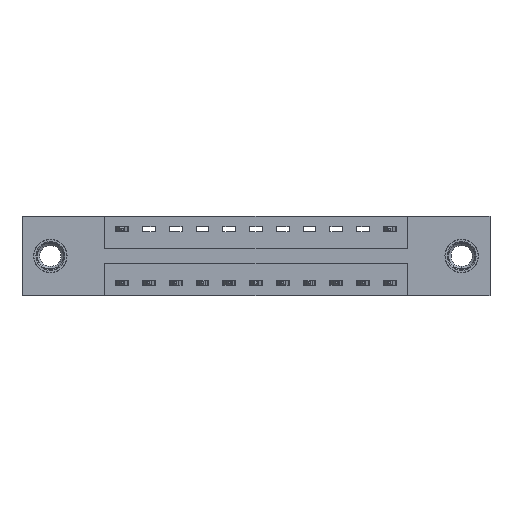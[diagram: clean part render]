
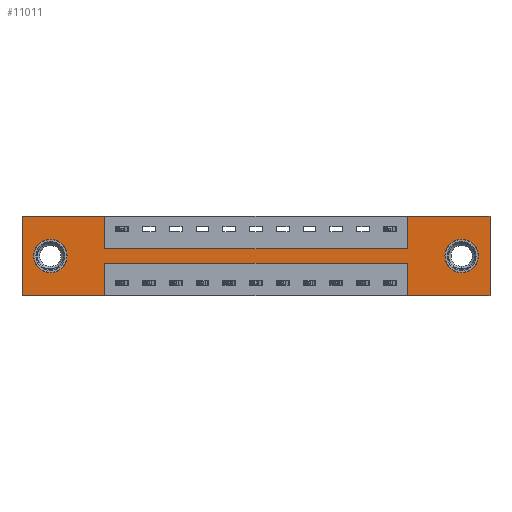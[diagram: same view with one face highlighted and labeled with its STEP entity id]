
A CAD part, front view. The second image highlights one B-rep face of the part: STEP entity #11011.
In plain terms, the highlighted planar face has unit normal (0, -1, 0).
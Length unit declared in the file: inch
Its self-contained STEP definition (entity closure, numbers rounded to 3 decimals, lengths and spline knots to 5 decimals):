
#6 = VECTOR ( 'NONE', #2793, 39.37008 ) ;
#59 = VERTEX_POINT ( 'NONE', #8711 ) ;
#99 = VERTEX_POINT ( 'NONE', #3134 ) ;
#326 = CARTESIAN_POINT ( 'NONE',  ( 0.3875, 0., -0.37 ) ) ;
#613 = VECTOR ( 'NONE', #11234, 39.37008 ) ;
#619 = VERTEX_POINT ( 'NONE', #6889 ) ;
#634 = CARTESIAN_POINT ( 'NONE',  ( 0.3875, 0., -0.15 ) ) ;
#767 = VECTOR ( 'NONE', #6159, 39.37008 ) ;
#859 = VERTEX_POINT ( 'NONE', #8142 ) ;
#861 = VECTOR ( 'NONE', #5536, 39.37008 ) ;
#1029 = CARTESIAN_POINT ( 'NONE',  ( 0.3875, 0., -0.37 ) ) ;
#1078 = VECTOR ( 'NONE', #11144, 39.37008 ) ;
#1171 = LINE ( 'NONE', #4607, #861 ) ;
#1278 = EDGE_CURVE ( 'NONE', #5420, #1296, #7348, .T. ) ;
#1296 = VERTEX_POINT ( 'NONE', #7767 ) ;
#1376 = FACE_BOUND ( 'NONE', #5382, .T. ) ;
#1487 = CIRCLE ( 'NONE', #11103, 0.078 ) ;
#1772 = CARTESIAN_POINT ( 'NONE',  ( 0.3875, 0., -0.22 ) ) ;
#1794 = LINE ( 'NONE', #8426, #11575 ) ;
#2146 = CARTESIAN_POINT ( 'NONE',  ( 2.0525, 0., -0.185 ) ) ;
#2613 = DIRECTION ( 'NONE',  ( 1., 0., 0. ) ) ;
#2614 = VECTOR ( 'NONE', #3877, 39.37008 ) ;
#2634 = VERTEX_POINT ( 'NONE', #5262 ) ;
#2656 = DIRECTION ( 'NONE',  ( 0., 1., 0. ) ) ;
#2790 = DIRECTION ( 'NONE',  ( 0., 0., 1. ) ) ;
#2793 = DIRECTION ( 'NONE',  ( -1., 0., 0. ) ) ;
#2811 = DIRECTION ( 'NONE',  ( 0., 0., 1. ) ) ;
#3043 = EDGE_LOOP ( 'NONE', ( #6996, #6897 ) ) ;
#3106 = DIRECTION ( 'NONE',  ( 0., 0., -1. ) ) ;
#3134 = CARTESIAN_POINT ( 'NONE',  ( 1.7975, 0., -0.15 ) ) ;
#3207 = LINE ( 'NONE', #10303, #613 ) ;
#3295 = EDGE_CURVE ( 'NONE', #4076, #99, #3652, .T. ) ;
#3652 = LINE ( 'NONE', #634, #5839 ) ;
#3877 = DIRECTION ( 'NONE',  ( 1., 0., 0. ) ) ;
#3961 = FACE_OUTER_BOUND ( 'NONE', #4950, .T. ) ;
#3971 = DIRECTION ( 'NONE',  ( 0., 0., -1. ) ) ;
#4076 = VERTEX_POINT ( 'NONE', #11130 ) ;
#4156 = LINE ( 'NONE', #8419, #11649 ) ;
#4180 = CARTESIAN_POINT ( 'NONE',  ( 2.0525, 0., -0.185 ) ) ;
#4206 = CARTESIAN_POINT ( 'NONE',  ( 2.0525, 0., -0.263 ) ) ;
#4257 = VECTOR ( 'NONE', #9504, 39.37008 ) ;
#4414 = EDGE_CURVE ( 'NONE', #1296, #5420, #10409, .T. ) ;
#4607 = CARTESIAN_POINT ( 'NONE',  ( 2.185, 0., 0. ) ) ;
#4625 = DIRECTION ( 'NONE',  ( 0., -1., 0. ) ) ;
#4796 = EDGE_CURVE ( 'NONE', #99, #59, #11270, .T. ) ;
#4950 = EDGE_LOOP ( 'NONE', ( #6749, #6699, #6639, #6567, #6296, #6274, #5981, #5965, #5869, #10560, #9883, #9823 ) ) ;
#4951 = AXIS2_PLACEMENT_3D ( 'NONE', #4180, #10756, #5116 ) ;
#5116 = DIRECTION ( 'NONE',  ( 0., 0., -1. ) ) ;
#5120 = LINE ( 'NONE', #6506, #6 ) ;
#5128 = EDGE_CURVE ( 'NONE', #6723, #7833, #5120, .T. ) ;
#5262 = CARTESIAN_POINT ( 'NONE',  ( 0.1325, 0., -0.107 ) ) ;
#5382 = EDGE_LOOP ( 'NONE', ( #7654, #7159 ) ) ;
#5420 = VERTEX_POINT ( 'NONE', #4206 ) ;
#5475 = CARTESIAN_POINT ( 'NONE',  ( 0.1325, 0., -0.185 ) ) ;
#5536 = DIRECTION ( 'NONE',  ( 0., 0., -1. ) ) ;
#5779 = VECTOR ( 'NONE', #3971, 39.37008 ) ;
#5786 = EDGE_CURVE ( 'NONE', #8634, #859, #1794, .T. ) ;
#5839 = VECTOR ( 'NONE', #2613, 39.37008 ) ;
#5869 = ORIENTED_EDGE ( 'NONE', *, *, #10586, .F. ) ;
#5879 = CARTESIAN_POINT ( 'NONE',  ( 0., 0., -0.37 ) ) ;
#5965 = ORIENTED_EDGE ( 'NONE', *, *, #3295, .F. ) ;
#5981 = ORIENTED_EDGE ( 'NONE', *, *, #4796, .F. ) ;
#6005 = AXIS2_PLACEMENT_3D ( 'NONE', #2146, #8724, #3106 ) ;
#6079 = LINE ( 'NONE', #1029, #5779 ) ;
#6159 = DIRECTION ( 'NONE',  ( -1., 0., 0. ) ) ;
#6274 = ORIENTED_EDGE ( 'NONE', *, *, #11682, .F. ) ;
#6284 = EDGE_CURVE ( 'NONE', #619, #2634, #1487, .T. ) ;
#6296 = ORIENTED_EDGE ( 'NONE', *, *, #7002, .F. ) ;
#6297 = CARTESIAN_POINT ( 'NONE',  ( 1.7975, 0., -0.37 ) ) ;
#6395 = DIRECTION ( 'NONE',  ( 0., 0., 1. ) ) ;
#6415 = CARTESIAN_POINT ( 'NONE',  ( 0.3875, 0., 0. ) ) ;
#6445 = PLANE ( 'NONE',  #9887 ) ;
#6506 = CARTESIAN_POINT ( 'NONE',  ( 0., 0., -0.37 ) ) ;
#6527 = EDGE_CURVE ( 'NONE', #9380, #6723, #6079, .T. ) ;
#6567 = ORIENTED_EDGE ( 'NONE', *, *, #11352, .F. ) ;
#6636 = CARTESIAN_POINT ( 'NONE',  ( 0.3875, 0., -0.22 ) ) ;
#6639 = ORIENTED_EDGE ( 'NONE', *, *, #11592, .F. ) ;
#6699 = ORIENTED_EDGE ( 'NONE', *, *, #11680, .F. ) ;
#6711 = LINE ( 'NONE', #6636, #4257 ) ;
#6723 = VERTEX_POINT ( 'NONE', #326 ) ;
#6749 = ORIENTED_EDGE ( 'NONE', *, *, #6527, .F. ) ;
#6889 = CARTESIAN_POINT ( 'NONE',  ( 0.1325, 0., -0.263 ) ) ;
#6897 = ORIENTED_EDGE ( 'NONE', *, *, #6284, .T. ) ;
#6918 = VERTEX_POINT ( 'NONE', #12002 ) ;
#6996 = ORIENTED_EDGE ( 'NONE', *, *, #12121, .T. ) ;
#7002 = EDGE_CURVE ( 'NONE', #11678, #8720, #1171, .T. ) ;
#7159 = ORIENTED_EDGE ( 'NONE', *, *, #1278, .T. ) ;
#7348 = CIRCLE ( 'NONE', #6005, 0.078 ) ;
#7654 = ORIENTED_EDGE ( 'NONE', *, *, #4414, .T. ) ;
#7767 = CARTESIAN_POINT ( 'NONE',  ( 2.0525, 0., -0.107 ) ) ;
#7833 = VERTEX_POINT ( 'NONE', #5879 ) ;
#8142 = CARTESIAN_POINT ( 'NONE',  ( 0.3875, 0., 0. ) ) ;
#8189 = CARTESIAN_POINT ( 'NONE',  ( 2.185, 0., -0.37 ) ) ;
#8262 = CARTESIAN_POINT ( 'NONE',  ( 0.1325, 0., -0.185 ) ) ;
#8333 = CARTESIAN_POINT ( 'NONE',  ( 0., 0., -0.37 ) ) ;
#8419 = CARTESIAN_POINT ( 'NONE',  ( 0., 0., 0. ) ) ;
#8426 = CARTESIAN_POINT ( 'NONE',  ( 0., 0., 0. ) ) ;
#8538 = CARTESIAN_POINT ( 'NONE',  ( 2.185, 0., 0. ) ) ;
#8634 = VERTEX_POINT ( 'NONE', #9030 ) ;
#8652 = LINE ( 'NONE', #6415, #1078 ) ;
#8711 = CARTESIAN_POINT ( 'NONE',  ( 1.7975, 0., 0. ) ) ;
#8720 = VERTEX_POINT ( 'NONE', #8189 ) ;
#8724 = DIRECTION ( 'NONE',  ( 0., 1., 0. ) ) ;
#9030 = CARTESIAN_POINT ( 'NONE',  ( 0., 0., 0. ) ) ;
#9164 = AXIS2_PLACEMENT_3D ( 'NONE', #8262, #2656, #9251 ) ;
#9231 = VERTEX_POINT ( 'NONE', #6297 ) ;
#9251 = DIRECTION ( 'NONE',  ( 0., 0., 1. ) ) ;
#9362 = VECTOR ( 'NONE', #2790, 39.37008 ) ;
#9380 = VERTEX_POINT ( 'NONE', #1772 ) ;
#9384 = CARTESIAN_POINT ( 'NONE',  ( 1.7975, 0., 0. ) ) ;
#9428 = EDGE_CURVE ( 'NONE', #7833, #8634, #4156, .T. ) ;
#9504 = DIRECTION ( 'NONE',  ( -1., 0., 0. ) ) ;
#9823 = ORIENTED_EDGE ( 'NONE', *, *, #5128, .F. ) ;
#9883 = ORIENTED_EDGE ( 'NONE', *, *, #9428, .F. ) ;
#9887 = AXIS2_PLACEMENT_3D ( 'NONE', #8333, #4625, #11207 ) ;
#9934 = CARTESIAN_POINT ( 'NONE',  ( 0., 0., -0.37 ) ) ;
#10303 = CARTESIAN_POINT ( 'NONE',  ( 1.7975, 0., -0.37 ) ) ;
#10409 = CIRCLE ( 'NONE', #4951, 0.078 ) ;
#10462 = CARTESIAN_POINT ( 'NONE',  ( 0., 0., 0. ) ) ;
#10560 = ORIENTED_EDGE ( 'NONE', *, *, #5786, .F. ) ;
#10586 = EDGE_CURVE ( 'NONE', #859, #4076, #8652, .T. ) ;
#10756 = DIRECTION ( 'NONE',  ( 0., 1., 0. ) ) ;
#10863 = CIRCLE ( 'NONE', #9164, 0.078 ) ;
#10886 = LINE ( 'NONE', #9934, #767 ) ;
#11011 = ADVANCED_FACE ( 'NONE', ( #1376, #11451, #3961 ), #6445, .T. ) ;
#11103 = AXIS2_PLACEMENT_3D ( 'NONE', #5475, #12061, #6395 ) ;
#11130 = CARTESIAN_POINT ( 'NONE',  ( 0.3875, 0., -0.15 ) ) ;
#11144 = DIRECTION ( 'NONE',  ( 0., 0., -1. ) ) ;
#11207 = DIRECTION ( 'NONE',  ( 0., 0., -1. ) ) ;
#11234 = DIRECTION ( 'NONE',  ( 0., 0., 1. ) ) ;
#11270 = LINE ( 'NONE', #9384, #9362 ) ;
#11352 = EDGE_CURVE ( 'NONE', #8720, #9231, #10886, .T. ) ;
#11451 = FACE_BOUND ( 'NONE', #3043, .T. ) ;
#11575 = VECTOR ( 'NONE', #12235, 39.37008 ) ;
#11592 = EDGE_CURVE ( 'NONE', #9231, #6918, #3207, .T. ) ;
#11649 = VECTOR ( 'NONE', #2811, 39.37008 ) ;
#11678 = VERTEX_POINT ( 'NONE', #8538 ) ;
#11680 = EDGE_CURVE ( 'NONE', #6918, #9380, #6711, .T. ) ;
#11682 = EDGE_CURVE ( 'NONE', #59, #11678, #11748, .T. ) ;
#11748 = LINE ( 'NONE', #10462, #2614 ) ;
#12002 = CARTESIAN_POINT ( 'NONE',  ( 1.7975, 0., -0.22 ) ) ;
#12061 = DIRECTION ( 'NONE',  ( 0., 1., 0. ) ) ;
#12121 = EDGE_CURVE ( 'NONE', #2634, #619, #10863, .T. ) ;
#12235 = DIRECTION ( 'NONE',  ( 1., 0., 0. ) ) ;
